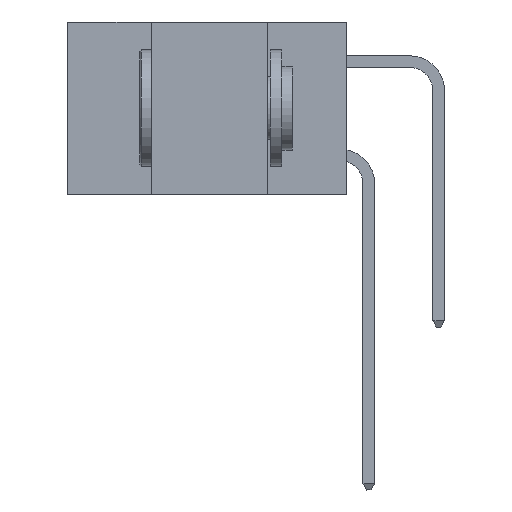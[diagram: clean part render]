
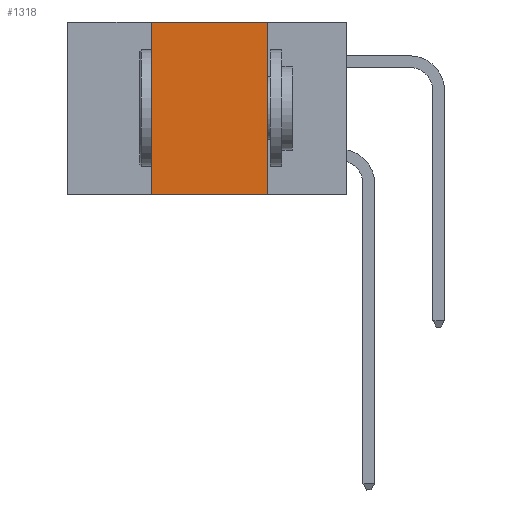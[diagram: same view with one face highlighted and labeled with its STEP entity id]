
A CAD part, left-side view. The second image highlights one B-rep face of the part: STEP entity #1318.
In plain terms, the highlighted planar face has unit normal (-1, 0, 0).
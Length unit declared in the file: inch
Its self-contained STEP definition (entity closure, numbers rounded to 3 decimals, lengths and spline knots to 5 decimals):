
#1133 = CARTESIAN_POINT ( 'NONE',  ( 0., 0.6, -0.37 ) ) ;
#1318 = ADVANCED_FACE ( 'NONE', ( #15363 ), #21209, .F. ) ;
#1510 = CARTESIAN_POINT ( 'NONE',  ( 0., 0.42, -0.37 ) ) ;
#2175 = VERTEX_POINT ( 'NONE', #1510 ) ;
#2237 = VECTOR ( 'NONE', #15156, 39.37008 ) ;
#2284 = ORIENTED_EDGE ( 'NONE', *, *, #11732, .F. ) ;
#2311 = VERTEX_POINT ( 'NONE', #6106 ) ;
#3093 = DIRECTION ( 'NONE',  ( 0., 0., 1. ) ) ;
#4285 = EDGE_CURVE ( 'NONE', #2175, #15555, #8049, .T. ) ;
#6106 = CARTESIAN_POINT ( 'NONE',  ( 0., 0.17, 0. ) ) ;
#6279 = DIRECTION ( 'NONE',  ( 0., 0., -1. ) ) ;
#6352 = CARTESIAN_POINT ( 'NONE',  ( 0., 0.17, 0. ) ) ;
#7524 = DIRECTION ( 'NONE',  ( 1., 0., 0. ) ) ;
#7631 = ORIENTED_EDGE ( 'NONE', *, *, #19794, .F. ) ;
#7999 = CARTESIAN_POINT ( 'NONE',  ( 0., 0.42, 0. ) ) ;
#8049 = LINE ( 'NONE', #1133, #2237 ) ;
#8922 = VECTOR ( 'NONE', #16627, 39.37008 ) ;
#9197 = LINE ( 'NONE', #13008, #8922 ) ;
#10619 = EDGE_LOOP ( 'NONE', ( #2284, #7631, #21141, #11792 ) ) ;
#11035 = CARTESIAN_POINT ( 'NONE',  ( 0., 0.17, -0.37 ) ) ;
#11636 = VECTOR ( 'NONE', #6279, 39.37008 ) ;
#11729 = CARTESIAN_POINT ( 'NONE',  ( 0., 0.42, 0. ) ) ;
#11732 = EDGE_CURVE ( 'NONE', #2311, #15555, #22250, .T. ) ;
#11792 = ORIENTED_EDGE ( 'NONE', *, *, #4285, .T. ) ;
#12400 = CARTESIAN_POINT ( 'NONE',  ( 0., 0.6, 0. ) ) ;
#13008 = CARTESIAN_POINT ( 'NONE',  ( 0., 0.6, 0. ) ) ;
#14588 = DIRECTION ( 'NONE',  ( 0., 0., -1. ) ) ;
#15156 = DIRECTION ( 'NONE',  ( 0., -1., 0. ) ) ;
#15363 = FACE_OUTER_BOUND ( 'NONE', #10619, .T. ) ;
#15555 = VERTEX_POINT ( 'NONE', #11035 ) ;
#16437 = VECTOR ( 'NONE', #3093, 39.37008 ) ;
#16627 = DIRECTION ( 'NONE',  ( 0., -1., 0. ) ) ;
#18895 = VERTEX_POINT ( 'NONE', #7999 ) ;
#19735 = LINE ( 'NONE', #11729, #16437 ) ;
#19794 = EDGE_CURVE ( 'NONE', #18895, #2311, #9197, .T. ) ;
#20413 = EDGE_CURVE ( 'NONE', #2175, #18895, #19735, .T. ) ;
#21141 = ORIENTED_EDGE ( 'NONE', *, *, #20413, .F. ) ;
#21209 = PLANE ( 'NONE',  #21785 ) ;
#21785 = AXIS2_PLACEMENT_3D ( 'NONE', #12400, #7524, #14588 ) ;
#22250 = LINE ( 'NONE', #6352, #11636 ) ;
